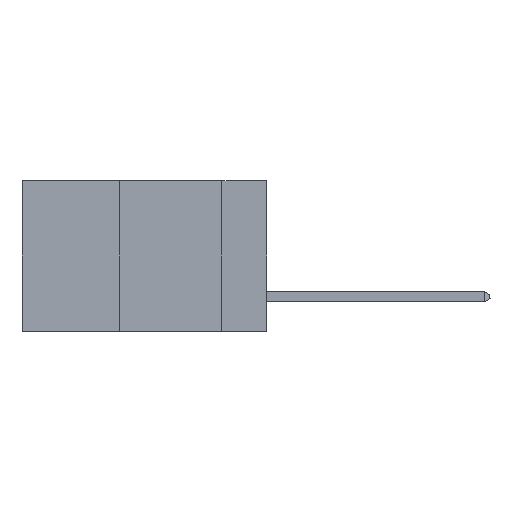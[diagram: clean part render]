
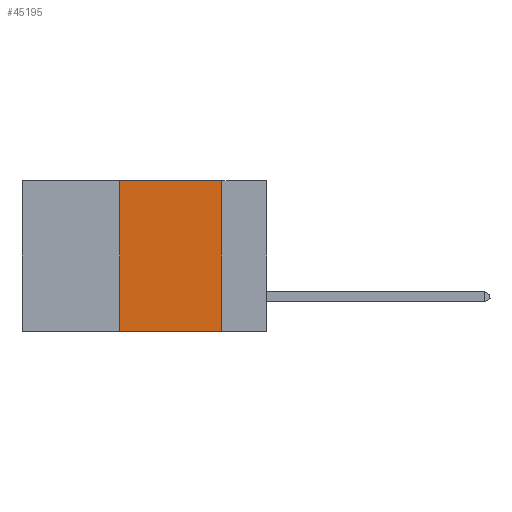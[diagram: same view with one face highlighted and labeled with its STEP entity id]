
A CAD part, left-side view. The second image highlights one B-rep face of the part: STEP entity #45195.
In plain terms, the highlighted planar face has unit normal (-1, 0, 0).
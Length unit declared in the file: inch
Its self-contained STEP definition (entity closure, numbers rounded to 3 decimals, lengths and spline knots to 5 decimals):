
#1231 = EDGE_CURVE ( 'NONE', #43072, #18078, #40646, .T. ) ;
#3670 = CARTESIAN_POINT ( 'NONE',  ( 0., 0.6, 0. ) ) ;
#3955 = EDGE_CURVE ( 'NONE', #42870, #18078, #44762, .T. ) ;
#5052 = VECTOR ( 'NONE', #17365, 39.37008 ) ;
#5136 = FACE_OUTER_BOUND ( 'NONE', #25676, .T. ) ;
#6316 = LINE ( 'NONE', #32414, #42485 ) ;
#8843 = CARTESIAN_POINT ( 'NONE',  ( 0., 0.36, 0. ) ) ;
#9183 = LINE ( 'NONE', #8843, #43089 ) ;
#11405 = ORIENTED_EDGE ( 'NONE', *, *, #24215, .F. ) ;
#11412 = DIRECTION ( 'NONE',  ( 0., -1., 0. ) ) ;
#11628 = CARTESIAN_POINT ( 'NONE',  ( 0., 0.36, 0. ) ) ;
#14066 = ORIENTED_EDGE ( 'NONE', *, *, #1231, .T. ) ;
#14886 = PLANE ( 'NONE',  #24343 ) ;
#17365 = DIRECTION ( 'NONE',  ( 0., -1., 0. ) ) ;
#18078 = VERTEX_POINT ( 'NONE', #23073 ) ;
#18606 = ORIENTED_EDGE ( 'NONE', *, *, #3955, .F. ) ;
#20077 = DIRECTION ( 'NONE',  ( 0., 0., -1. ) ) ;
#23073 = CARTESIAN_POINT ( 'NONE',  ( 0., 0.11, -0.37 ) ) ;
#24215 = EDGE_CURVE ( 'NONE', #43072, #32769, #9183, .T. ) ;
#24343 = AXIS2_PLACEMENT_3D ( 'NONE', #3670, #36586, #43864 ) ;
#25676 = EDGE_LOOP ( 'NONE', ( #18606, #41425, #11405, #14066 ) ) ;
#32414 = CARTESIAN_POINT ( 'NONE',  ( 0., 0.6, 0. ) ) ;
#32769 = VERTEX_POINT ( 'NONE', #11628 ) ;
#34182 = CARTESIAN_POINT ( 'NONE',  ( 0., 0.11, 0. ) ) ;
#35515 = CARTESIAN_POINT ( 'NONE',  ( 0., 0.11, 0. ) ) ;
#35812 = CARTESIAN_POINT ( 'NONE',  ( 0., 0.36, -0.37 ) ) ;
#36586 = DIRECTION ( 'NONE',  ( 1., 0., 0. ) ) ;
#38350 = CARTESIAN_POINT ( 'NONE',  ( 0., 0.6, -0.37 ) ) ;
#40646 = LINE ( 'NONE', #38350, #5052 ) ;
#41425 = ORIENTED_EDGE ( 'NONE', *, *, #44595, .F. ) ;
#42485 = VECTOR ( 'NONE', #11412, 39.37008 ) ;
#42870 = VERTEX_POINT ( 'NONE', #35515 ) ;
#43072 = VERTEX_POINT ( 'NONE', #35812 ) ;
#43089 = VECTOR ( 'NONE', #43389, 39.37008 ) ;
#43389 = DIRECTION ( 'NONE',  ( 0., 0., 1. ) ) ;
#43864 = DIRECTION ( 'NONE',  ( 0., 0., -1. ) ) ;
#44595 = EDGE_CURVE ( 'NONE', #32769, #42870, #6316, .T. ) ;
#44762 = LINE ( 'NONE', #34182, #45325 ) ;
#45195 = ADVANCED_FACE ( 'NONE', ( #5136 ), #14886, .F. ) ;
#45325 = VECTOR ( 'NONE', #20077, 39.37008 ) ;
